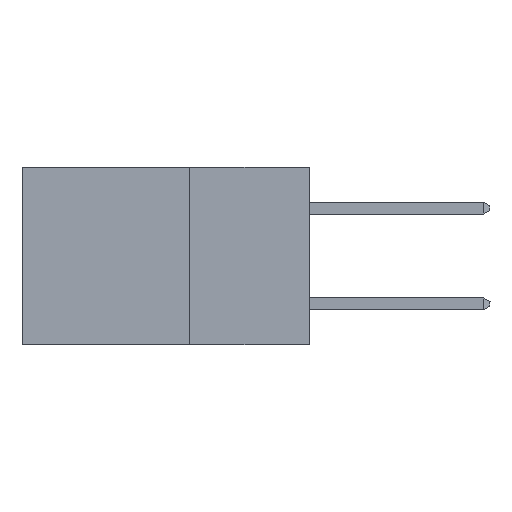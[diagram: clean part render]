
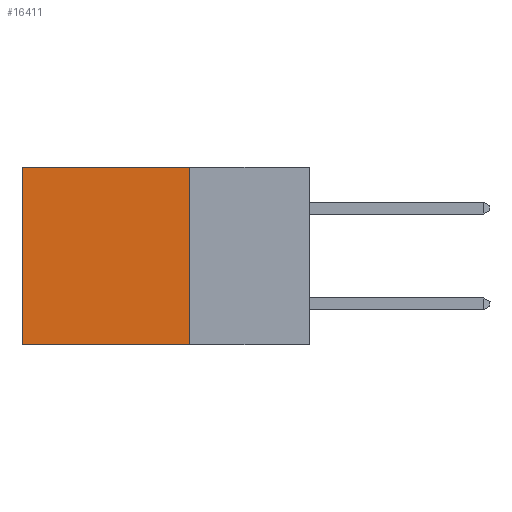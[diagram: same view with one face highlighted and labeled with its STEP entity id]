
A CAD part, left-side view. The second image highlights one B-rep face of the part: STEP entity #16411.
In plain terms, the highlighted planar face has unit normal (-1, 0, 0).
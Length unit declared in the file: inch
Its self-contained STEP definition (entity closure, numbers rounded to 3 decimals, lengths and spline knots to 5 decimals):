
#584 = EDGE_CURVE ( 'NONE', #18198, #7310, #41491, .T. ) ;
#896 = EDGE_CURVE ( 'NONE', #21794, #18198, #37647, .T. ) ;
#4651 = DIRECTION ( 'NONE',  ( 0., 1., 0. ) ) ;
#6039 = CARTESIAN_POINT ( 'NONE',  ( 0.2875, 0.25, -0.37 ) ) ;
#7310 = VERTEX_POINT ( 'NONE', #16763 ) ;
#7615 = VECTOR ( 'NONE', #4651, 39.37008 ) ;
#9147 = CARTESIAN_POINT ( 'NONE',  ( 0.2875, 0.25, 0. ) ) ;
#9372 = CARTESIAN_POINT ( 'NONE',  ( 0.2875, 0.25, 0. ) ) ;
#9969 = CARTESIAN_POINT ( 'NONE',  ( 0.2875, 0.25, -0.37 ) ) ;
#10130 = ORIENTED_EDGE ( 'NONE', *, *, #21818, .F. ) ;
#11838 = LINE ( 'NONE', #6039, #38716 ) ;
#13625 = LINE ( 'NONE', #9147, #24383 ) ;
#16411 = ADVANCED_FACE ( 'NONE', ( #35456 ), #29907, .F. ) ;
#16731 = DIRECTION ( 'NONE',  ( 0., 0., -1. ) ) ;
#16763 = CARTESIAN_POINT ( 'NONE',  ( 0.2875, 0.6, -0.37 ) ) ;
#18198 = VERTEX_POINT ( 'NONE', #24858 ) ;
#18266 = ORIENTED_EDGE ( 'NONE', *, *, #896, .T. ) ;
#18346 = ORIENTED_EDGE ( 'NONE', *, *, #29053, .F. ) ;
#21794 = VERTEX_POINT ( 'NONE', #22646 ) ;
#21818 = EDGE_CURVE ( 'NONE', #21794, #39012, #13625, .T. ) ;
#22353 = DIRECTION ( 'NONE',  ( 0., 0., -1. ) ) ;
#22646 = CARTESIAN_POINT ( 'NONE',  ( 0.2875, 0.25, 0. ) ) ;
#22672 = VECTOR ( 'NONE', #44438, 39.37008 ) ;
#24383 = VECTOR ( 'NONE', #22353, 39.37008 ) ;
#24858 = CARTESIAN_POINT ( 'NONE',  ( 0.2875, 0.6, 0. ) ) ;
#29053 = EDGE_CURVE ( 'NONE', #39012, #7310, #11838, .T. ) ;
#29907 = PLANE ( 'NONE',  #37881 ) ;
#35456 = FACE_OUTER_BOUND ( 'NONE', #36578, .T. ) ;
#36539 = ORIENTED_EDGE ( 'NONE', *, *, #584, .T. ) ;
#36578 = EDGE_LOOP ( 'NONE', ( #36539, #18346, #10130, #18266 ) ) ;
#36968 = CARTESIAN_POINT ( 'NONE',  ( 0.2875, 0.6, 0. ) ) ;
#37647 = LINE ( 'NONE', #42513, #7615 ) ;
#37881 = AXIS2_PLACEMENT_3D ( 'NONE', #9372, #40303, #16731 ) ;
#38716 = VECTOR ( 'NONE', #43945, 39.37008 ) ;
#39012 = VERTEX_POINT ( 'NONE', #9969 ) ;
#40303 = DIRECTION ( 'NONE',  ( 1., 0., 0. ) ) ;
#41491 = LINE ( 'NONE', #36968, #22672 ) ;
#42513 = CARTESIAN_POINT ( 'NONE',  ( 0.2875, 0.25, 0. ) ) ;
#43945 = DIRECTION ( 'NONE',  ( 0., 1., 0. ) ) ;
#44438 = DIRECTION ( 'NONE',  ( 0., 0., -1. ) ) ;
